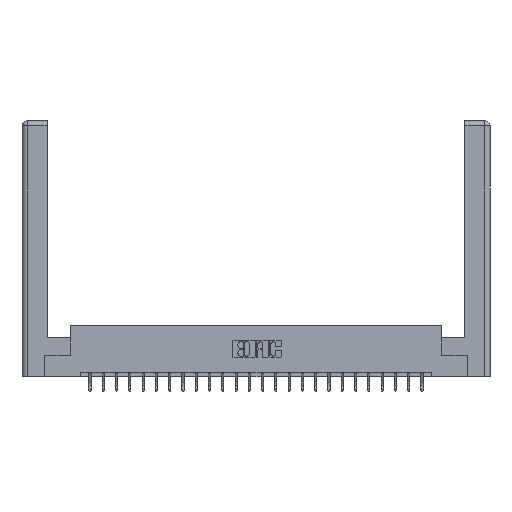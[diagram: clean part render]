
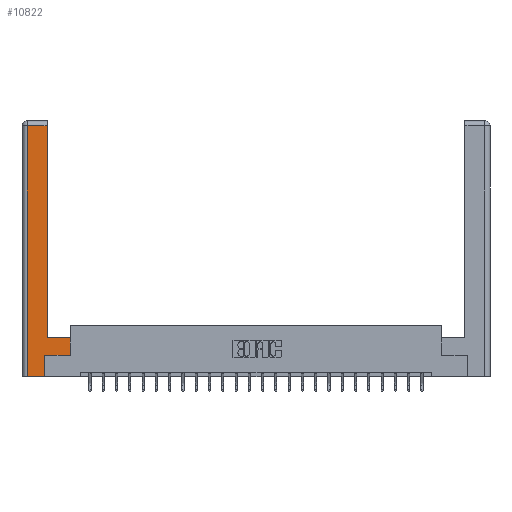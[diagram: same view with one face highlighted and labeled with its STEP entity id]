
A CAD part, top view. The second image highlights one B-rep face of the part: STEP entity #10822.
In plain terms, the highlighted planar face has unit normal (0, 0, 1).
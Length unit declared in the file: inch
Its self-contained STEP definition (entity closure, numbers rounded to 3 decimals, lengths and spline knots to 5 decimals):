
#49 = CARTESIAN_POINT ( 'NONE',  ( 0.565, 0.245, 0. ) ) ;
#668 = LINE ( 'NONE', #8847, #18562 ) ;
#725 = VECTOR ( 'NONE', #22545, 39.37008 ) ;
#1388 = CARTESIAN_POINT ( 'NONE',  ( 0.565, 0.245, 0. ) ) ;
#1406 = VECTOR ( 'NONE', #23982, 39.37008 ) ;
#1433 = ORIENTED_EDGE ( 'NONE', *, *, #23925, .T. ) ;
#1434 = VECTOR ( 'NONE', #16279, 39.37008 ) ;
#1967 = VERTEX_POINT ( 'NONE', #6767 ) ;
#3008 = CARTESIAN_POINT ( 'NONE',  ( 0.295, 0.45, 0. ) ) ;
#3034 = CARTESIAN_POINT ( 'NONE',  ( 0.0615, 0., 0. ) ) ;
#3195 = VERTEX_POINT ( 'NONE', #18942 ) ;
#3439 = CARTESIAN_POINT ( 'NONE',  ( 0.265, 0.245, 0. ) ) ;
#3583 = CARTESIAN_POINT ( 'NONE',  ( 0.295, 3., 0. ) ) ;
#4672 = EDGE_CURVE ( 'NONE', #20500, #13588, #10092, .T. ) ;
#5318 = ORIENTED_EDGE ( 'NONE', *, *, #12028, .T. ) ;
#5394 = DIRECTION ( 'NONE',  ( 0., 1., 0. ) ) ;
#5527 = CARTESIAN_POINT ( 'NONE',  ( 0., 0., 0. ) ) ;
#5834 = ORIENTED_EDGE ( 'NONE', *, *, #8593, .T. ) ;
#6767 = CARTESIAN_POINT ( 'NONE',  ( 0.295, 0.45, 0. ) ) ;
#7019 = FACE_OUTER_BOUND ( 'NONE', #22757, .T. ) ;
#7148 = DIRECTION ( 'NONE',  ( 0., -1., 0. ) ) ;
#7220 = CARTESIAN_POINT ( 'NONE',  ( 0.565, 0.45, 0. ) ) ;
#7322 = VERTEX_POINT ( 'NONE', #13402 ) ;
#7458 = DIRECTION ( 'NONE',  ( 0., 0., -1. ) ) ;
#8573 = CARTESIAN_POINT ( 'NONE',  ( 0.0615, 2.94, 0. ) ) ;
#8593 = EDGE_CURVE ( 'NONE', #13588, #12069, #20515, .T. ) ;
#8761 = EDGE_CURVE ( 'NONE', #20678, #20500, #14460, .T. ) ;
#8836 = EDGE_CURVE ( 'NONE', #3195, #7322, #9603, .T. ) ;
#8847 = CARTESIAN_POINT ( 'NONE',  ( 0.0615, 0., 0. ) ) ;
#9247 = VERTEX_POINT ( 'NONE', #23745 ) ;
#9409 = DIRECTION ( 'NONE',  ( -1., 0., 0. ) ) ;
#9526 = VECTOR ( 'NONE', #5394, 39.37008 ) ;
#9603 = LINE ( 'NONE', #8573, #1406 ) ;
#9941 = VECTOR ( 'NONE', #22728, 39.37008 ) ;
#9980 = DIRECTION ( 'NONE',  ( 1., 0., 0. ) ) ;
#10092 = LINE ( 'NONE', #3439, #9526 ) ;
#10822 = ADVANCED_FACE ( 'NONE', ( #7019 ), #17101, .F. ) ;
#11403 = ORIENTED_EDGE ( 'NONE', *, *, #4672, .T. ) ;
#12028 = EDGE_CURVE ( 'NONE', #1967, #3195, #16005, .T. ) ;
#12069 = VERTEX_POINT ( 'NONE', #1388 ) ;
#12182 = ORIENTED_EDGE ( 'NONE', *, *, #8836, .T. ) ;
#12623 = ORIENTED_EDGE ( 'NONE', *, *, #18012, .T. ) ;
#13402 = CARTESIAN_POINT ( 'NONE',  ( 0.0615, 2.94, 0. ) ) ;
#13588 = VERTEX_POINT ( 'NONE', #19405 ) ;
#14079 = LINE ( 'NONE', #7220, #725 ) ;
#14124 = CARTESIAN_POINT ( 'NONE',  ( 0.265, 0., 0. ) ) ;
#14460 = LINE ( 'NONE', #21799, #1434 ) ;
#14575 = ORIENTED_EDGE ( 'NONE', *, *, #8761, .T. ) ;
#14887 = LINE ( 'NONE', #3008, #16975 ) ;
#15752 = ORIENTED_EDGE ( 'NONE', *, *, #18971, .T. ) ;
#16005 = LINE ( 'NONE', #3583, #9941 ) ;
#16279 = DIRECTION ( 'NONE',  ( 1., 0., 0. ) ) ;
#16975 = VECTOR ( 'NONE', #18080, 39.37008 ) ;
#17101 = PLANE ( 'NONE',  #17423 ) ;
#17423 = AXIS2_PLACEMENT_3D ( 'NONE', #5527, #7458, #9409 ) ;
#18012 = EDGE_CURVE ( 'NONE', #7322, #20678, #668, .T. ) ;
#18080 = DIRECTION ( 'NONE',  ( -1., 0., 0. ) ) ;
#18562 = VECTOR ( 'NONE', #7148, 39.37008 ) ;
#18942 = CARTESIAN_POINT ( 'NONE',  ( 0.295, 2.94, 0. ) ) ;
#18971 = EDGE_CURVE ( 'NONE', #9247, #1967, #14887, .T. ) ;
#19405 = CARTESIAN_POINT ( 'NONE',  ( 0.265, 0.245, 0. ) ) ;
#20206 = VECTOR ( 'NONE', #9980, 39.37008 ) ;
#20500 = VERTEX_POINT ( 'NONE', #14124 ) ;
#20515 = LINE ( 'NONE', #49, #20206 ) ;
#20678 = VERTEX_POINT ( 'NONE', #3034 ) ;
#21799 = CARTESIAN_POINT ( 'NONE',  ( 0.265, 0., 0. ) ) ;
#22545 = DIRECTION ( 'NONE',  ( 0., 1., 0. ) ) ;
#22728 = DIRECTION ( 'NONE',  ( 0., 1., 0. ) ) ;
#22757 = EDGE_LOOP ( 'NONE', ( #5318, #12182, #12623, #14575, #11403, #5834, #1433, #15752 ) ) ;
#23745 = CARTESIAN_POINT ( 'NONE',  ( 0.565, 0.45, 0. ) ) ;
#23925 = EDGE_CURVE ( 'NONE', #12069, #9247, #14079, .T. ) ;
#23982 = DIRECTION ( 'NONE',  ( -1., 0., 0. ) ) ;
